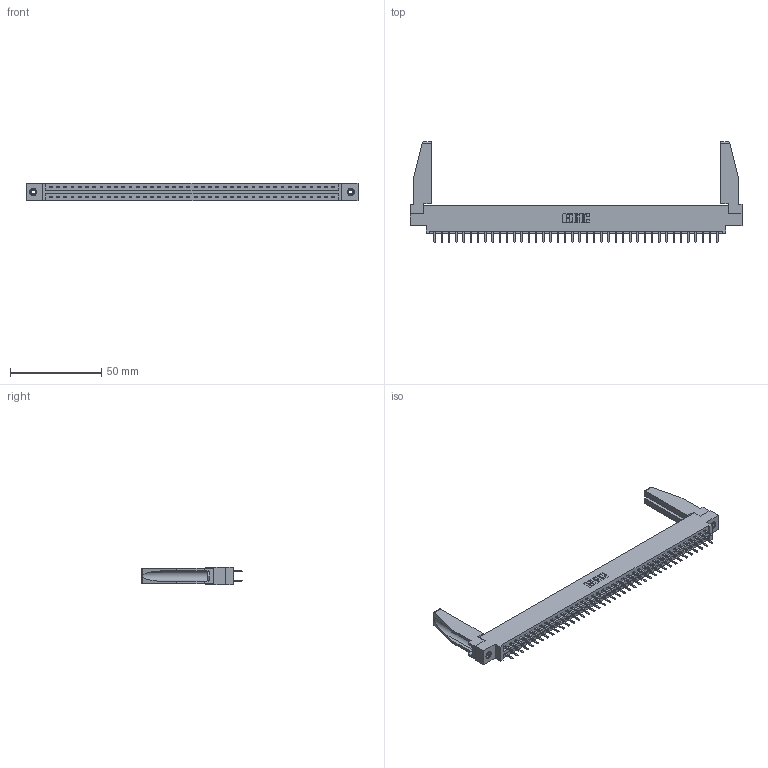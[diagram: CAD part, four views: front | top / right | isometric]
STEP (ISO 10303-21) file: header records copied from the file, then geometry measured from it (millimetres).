
FILE_DESCRIPTION (( 'STEP AP203' ), '1' );
FILE_NAME ('337-080-520-878.STEP', '2019-10-15T15:00:41', ( '' ), ( '' ), 'SwSTEP 2.0', 'SolidWorks 2016', '' );
FILE_SCHEMA (( 'CONFIG_CONTROL_DESIGN' ));
Length unit declared in the file: inch
Products named in the file (5): 345-292-001_345-293-120; 307-220-078; 337 Part_0.170 Offset - 0.156 Dia-TI; 345-250-001_345-250-001-102; 337-080-520-878
Assembly tree (85 placements, depth 2):
  337-080-520-878
    337 Part_0.170 Offset - 0.156 Dia-TI
    345-292-001_345-293-120  x80
    345-250-001_345-250-001-102  x2
    307-220-078  x2
Bounding box: 181.51 x 54.82 x 9.4 mm (x, y, z)
Volume: 22942.8 mm3; surface area: 25241 mm2
Topology: 85 solids, 85 shells, 4888 faces, 14173 edges, 9226 vertices
Faces by surface type: plane 3358, cylinder 1514, cone 12, torus 4
Entity records: 33958 total; most frequent: CARTESIAN_POINT 5736, ORIENTED_EDGE 5616, DIRECTION 4876, EDGE_CURVE 2808, LINE 2638, VECTOR 2638, VERTEX_POINT 1864, AXIS2_PLACEMENT_3D 1119
